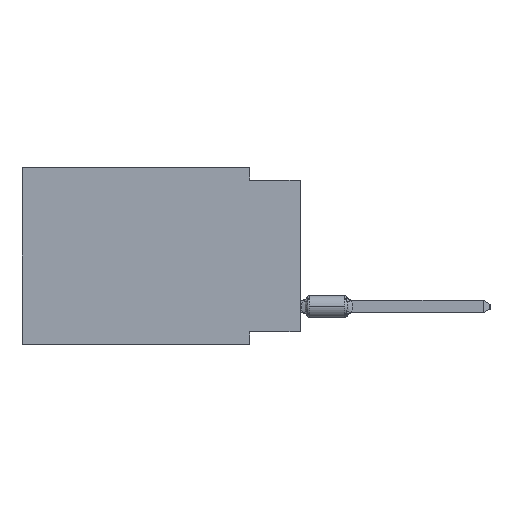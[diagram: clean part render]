
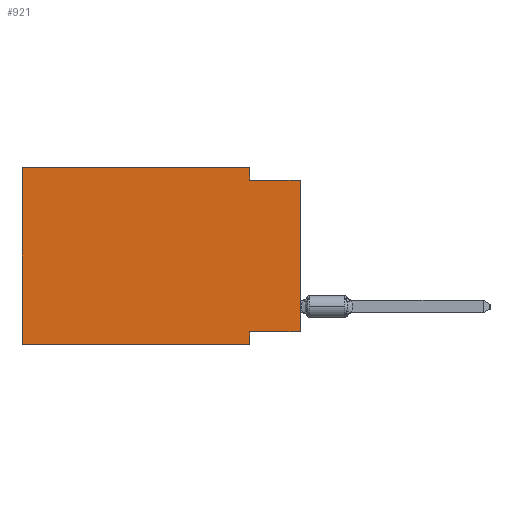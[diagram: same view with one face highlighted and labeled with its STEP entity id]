
A CAD part, left-side view. The second image highlights one B-rep face of the part: STEP entity #921.
In plain terms, the highlighted planar face has unit normal (-1, 0, 0).
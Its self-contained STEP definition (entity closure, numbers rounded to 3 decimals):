
#98 = DIRECTION ( 'NONE',  ( 0., 1., 0. ) ) ;
#365 = VERTEX_POINT ( 'NONE', #23913 ) ;
#884 = VECTOR ( 'NONE', #17373, 1000. ) ;
#921 = ADVANCED_FACE ( 'NONE', ( #26244 ), #30567, .F. ) ;
#1677 = VERTEX_POINT ( 'NONE', #11384 ) ;
#1904 = DIRECTION ( 'NONE',  ( 0., 0., -1. ) ) ;
#2036 = ORIENTED_EDGE ( 'NONE', *, *, #21575, .F. ) ;
#2072 = CARTESIAN_POINT ( 'NONE',  ( 0., 13.97, 0. ) ) ;
#3487 = VERTEX_POINT ( 'NONE', #12292 ) ;
#3947 = CARTESIAN_POINT ( 'NONE',  ( 0., 13.97, 0. ) ) ;
#4417 = EDGE_CURVE ( 'NONE', #30829, #27818, #24060, .T. ) ;
#5025 = VECTOR ( 'NONE', #21657, 1000. ) ;
#5790 = CARTESIAN_POINT ( 'NONE',  ( 0., 2.54, -8.89 ) ) ;
#6281 = EDGE_CURVE ( 'NONE', #365, #14781, #22321, .T. ) ;
#6524 = DIRECTION ( 'NONE',  ( 1., 0., 0. ) ) ;
#7837 = EDGE_CURVE ( 'NONE', #16643, #3487, #11952, .T. ) ;
#8937 = ORIENTED_EDGE ( 'NONE', *, *, #4417, .F. ) ;
#9268 = VECTOR ( 'NONE', #13291, 1000. ) ;
#9331 = CARTESIAN_POINT ( 'NONE',  ( 0., 0., -8.255 ) ) ;
#10008 = EDGE_CURVE ( 'NONE', #16643, #15112, #15019, .T. ) ;
#11370 = LINE ( 'NONE', #25383, #9268 ) ;
#11384 = CARTESIAN_POINT ( 'NONE',  ( 0., 2.54, -8.255 ) ) ;
#11415 = LINE ( 'NONE', #3947, #28582 ) ;
#11506 = CARTESIAN_POINT ( 'NONE',  ( 0., 2.54, -0.635 ) ) ;
#11530 = ORIENTED_EDGE ( 'NONE', *, *, #12992, .F. ) ;
#11952 = LINE ( 'NONE', #30315, #5025 ) ;
#12066 = CARTESIAN_POINT ( 'NONE',  ( 0., 13.97, 0. ) ) ;
#12292 = CARTESIAN_POINT ( 'NONE',  ( 0., 2.54, -8.89 ) ) ;
#12680 = EDGE_CURVE ( 'NONE', #365, #1677, #16799, .T. ) ;
#12992 = EDGE_CURVE ( 'NONE', #27818, #14781, #11370, .T. ) ;
#13291 = DIRECTION ( 'NONE',  ( 0., -1., 0. ) ) ;
#14113 = VECTOR ( 'NONE', #29440, 1000. ) ;
#14781 = VERTEX_POINT ( 'NONE', #19577 ) ;
#14952 = CARTESIAN_POINT ( 'NONE',  ( 0., 2.54, 0. ) ) ;
#15019 = LINE ( 'NONE', #19808, #24346 ) ;
#15112 = VERTEX_POINT ( 'NONE', #12066 ) ;
#16643 = VERTEX_POINT ( 'NONE', #16756 ) ;
#16756 = CARTESIAN_POINT ( 'NONE',  ( 0., 13.97, -8.89 ) ) ;
#16799 = LINE ( 'NONE', #9331, #30081 ) ;
#17063 = DIRECTION ( 'NONE',  ( 0., 0., 1. ) ) ;
#17196 = ORIENTED_EDGE ( 'NONE', *, *, #12680, .F. ) ;
#17202 = CARTESIAN_POINT ( 'NONE',  ( 0., 2.54, 0. ) ) ;
#17229 = CARTESIAN_POINT ( 'NONE',  ( 0., 0., 0. ) ) ;
#17373 = DIRECTION ( 'NONE',  ( 0., 0., -1. ) ) ;
#19018 = ORIENTED_EDGE ( 'NONE', *, *, #6281, .T. ) ;
#19414 = VECTOR ( 'NONE', #17063, 1000. ) ;
#19577 = CARTESIAN_POINT ( 'NONE',  ( 0., 0., -0.635 ) ) ;
#19808 = CARTESIAN_POINT ( 'NONE',  ( 0., 13.97, 0. ) ) ;
#21575 = EDGE_CURVE ( 'NONE', #15112, #30829, #11415, .T. ) ;
#21657 = DIRECTION ( 'NONE',  ( 0., -1., 0. ) ) ;
#22321 = LINE ( 'NONE', #17229, #19414 ) ;
#22649 = LINE ( 'NONE', #5790, #14113 ) ;
#22661 = DIRECTION ( 'NONE',  ( 0., 0., 1. ) ) ;
#23294 = AXIS2_PLACEMENT_3D ( 'NONE', #2072, #6524, #1904 ) ;
#23913 = CARTESIAN_POINT ( 'NONE',  ( 0., 0., -8.255 ) ) ;
#24060 = LINE ( 'NONE', #17202, #884 ) ;
#24346 = VECTOR ( 'NONE', #22661, 1000. ) ;
#25383 = CARTESIAN_POINT ( 'NONE',  ( 0., 0., -0.635 ) ) ;
#25743 = ORIENTED_EDGE ( 'NONE', *, *, #7837, .T. ) ;
#26244 = FACE_OUTER_BOUND ( 'NONE', #28321, .T. ) ;
#27410 = ORIENTED_EDGE ( 'NONE', *, *, #10008, .F. ) ;
#27531 = EDGE_CURVE ( 'NONE', #1677, #3487, #22649, .T. ) ;
#27671 = ORIENTED_EDGE ( 'NONE', *, *, #27531, .F. ) ;
#27818 = VERTEX_POINT ( 'NONE', #11506 ) ;
#28321 = EDGE_LOOP ( 'NONE', ( #19018, #11530, #8937, #2036, #27410, #25743, #27671, #17196 ) ) ;
#28445 = DIRECTION ( 'NONE',  ( 0., -1., 0. ) ) ;
#28582 = VECTOR ( 'NONE', #28445, 1000. ) ;
#29440 = DIRECTION ( 'NONE',  ( 0., 0., -1. ) ) ;
#30081 = VECTOR ( 'NONE', #98, 1000. ) ;
#30315 = CARTESIAN_POINT ( 'NONE',  ( 0., 13.97, -8.89 ) ) ;
#30567 = PLANE ( 'NONE',  #23294 ) ;
#30829 = VERTEX_POINT ( 'NONE', #14952 ) ;
